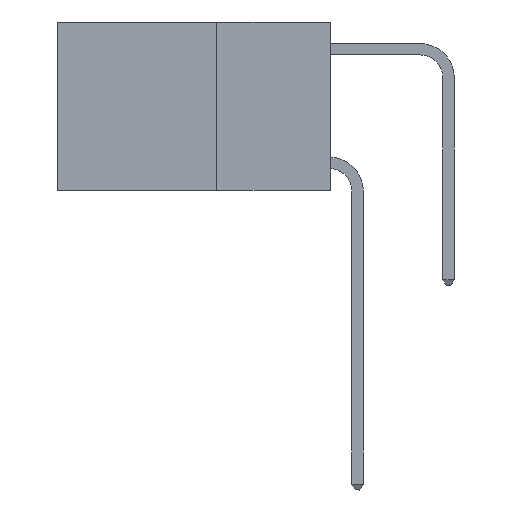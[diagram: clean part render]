
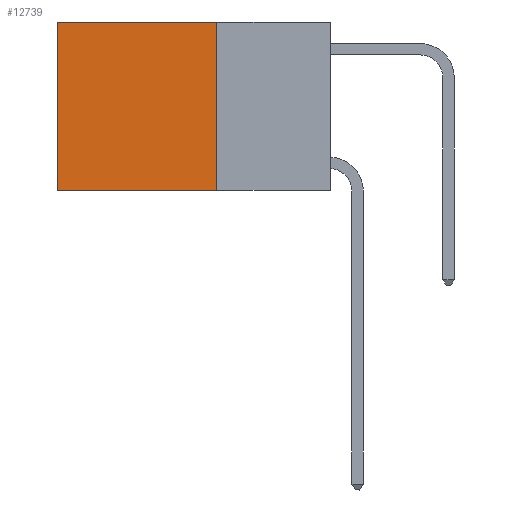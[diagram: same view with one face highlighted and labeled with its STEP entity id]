
A CAD part, left-side view. The second image highlights one B-rep face of the part: STEP entity #12739.
In plain terms, the highlighted planar face has unit normal (-1, 0, 0).
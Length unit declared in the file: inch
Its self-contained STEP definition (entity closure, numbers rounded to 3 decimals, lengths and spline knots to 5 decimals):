
#26 = VERTEX_POINT ( 'NONE', #10689 ) ;
#191 = VECTOR ( 'NONE', #4953, 39.37008 ) ;
#327 = VERTEX_POINT ( 'NONE', #1050 ) ;
#418 = DIRECTION ( 'NONE',  ( 0., 0., -1. ) ) ;
#421 = CARTESIAN_POINT ( 'NONE',  ( 0.2625, 0.6, -0.37 ) ) ;
#876 = EDGE_CURVE ( 'NONE', #26, #7844, #12108, .T. ) ;
#1050 = CARTESIAN_POINT ( 'NONE',  ( 0.2625, 0.25, -0.37 ) ) ;
#1154 = EDGE_LOOP ( 'NONE', ( #5723, #6922, #5452, #7145 ) ) ;
#2642 = VECTOR ( 'NONE', #418, 39.37008 ) ;
#2961 = DIRECTION ( 'NONE',  ( 0., 0., -1. ) ) ;
#3635 = FACE_OUTER_BOUND ( 'NONE', #1154, .T. ) ;
#4253 = CARTESIAN_POINT ( 'NONE',  ( 0.2625, 0.25, -0.37 ) ) ;
#4847 = EDGE_CURVE ( 'NONE', #6982, #26, #5432, .T. ) ;
#4953 = DIRECTION ( 'NONE',  ( 0., 1., 0. ) ) ;
#5331 = CARTESIAN_POINT ( 'NONE',  ( 0.2625, 0.25, 0. ) ) ;
#5432 = LINE ( 'NONE', #9759, #191 ) ;
#5452 = ORIENTED_EDGE ( 'NONE', *, *, #6009, .F. ) ;
#5626 = CARTESIAN_POINT ( 'NONE',  ( 0.2625, 0.25, 0. ) ) ;
#5723 = ORIENTED_EDGE ( 'NONE', *, *, #876, .T. ) ;
#6009 = EDGE_CURVE ( 'NONE', #6982, #327, #10507, .T. ) ;
#6028 = CARTESIAN_POINT ( 'NONE',  ( 0.2625, 0.25, 0. ) ) ;
#6922 = ORIENTED_EDGE ( 'NONE', *, *, #9439, .F. ) ;
#6982 = VERTEX_POINT ( 'NONE', #5331 ) ;
#7018 = DIRECTION ( 'NONE',  ( 0., 0., -1. ) ) ;
#7101 = VECTOR ( 'NONE', #2961, 39.37008 ) ;
#7145 = ORIENTED_EDGE ( 'NONE', *, *, #4847, .T. ) ;
#7274 = DIRECTION ( 'NONE',  ( 0., 1., 0. ) ) ;
#7844 = VERTEX_POINT ( 'NONE', #421 ) ;
#8139 = LINE ( 'NONE', #4253, #9984 ) ;
#8797 = AXIS2_PLACEMENT_3D ( 'NONE', #6028, #12637, #7018 ) ;
#9439 = EDGE_CURVE ( 'NONE', #327, #7844, #8139, .T. ) ;
#9759 = CARTESIAN_POINT ( 'NONE',  ( 0.2625, 0.25, 0. ) ) ;
#9984 = VECTOR ( 'NONE', #7274, 39.37008 ) ;
#10507 = LINE ( 'NONE', #5626, #2642 ) ;
#10526 = CARTESIAN_POINT ( 'NONE',  ( 0.2625, 0.6, 0. ) ) ;
#10689 = CARTESIAN_POINT ( 'NONE',  ( 0.2625, 0.6, 0. ) ) ;
#10727 = PLANE ( 'NONE',  #8797 ) ;
#12108 = LINE ( 'NONE', #10526, #7101 ) ;
#12637 = DIRECTION ( 'NONE',  ( 1., 0., 0. ) ) ;
#12739 = ADVANCED_FACE ( 'NONE', ( #3635 ), #10727, .F. ) ;
